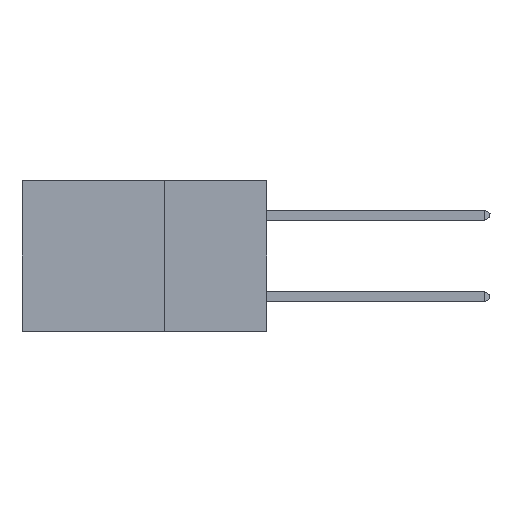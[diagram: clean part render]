
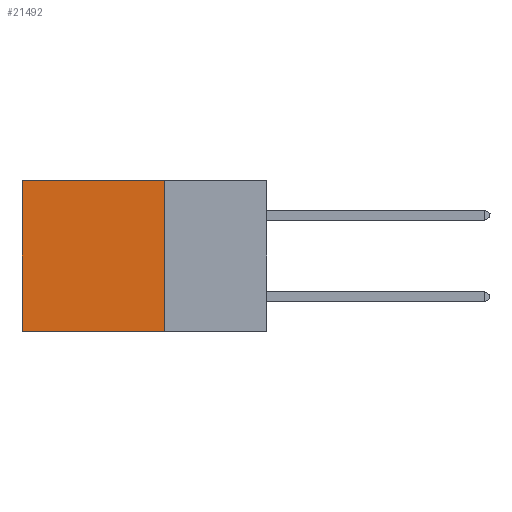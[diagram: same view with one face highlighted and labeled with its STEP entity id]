
A CAD part, left-side view. The second image highlights one B-rep face of the part: STEP entity #21492.
In plain terms, the highlighted planar face has unit normal (-1, 0, 0).
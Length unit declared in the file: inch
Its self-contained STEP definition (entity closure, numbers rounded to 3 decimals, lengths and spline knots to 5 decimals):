
#578 = CARTESIAN_POINT ( 'NONE',  ( 0.2875, 0.6, 0. ) ) ;
#723 = DIRECTION ( 'NONE',  ( 0., 0., -1. ) ) ;
#856 = PLANE ( 'NONE',  #13814 ) ;
#1374 = CARTESIAN_POINT ( 'NONE',  ( 0.2875, 0.6, 0. ) ) ;
#1841 = ORIENTED_EDGE ( 'NONE', *, *, #5590, .F. ) ;
#2267 = ORIENTED_EDGE ( 'NONE', *, *, #13636, .F. ) ;
#2281 = CARTESIAN_POINT ( 'NONE',  ( 0.2875, 0.25, -0.37 ) ) ;
#2628 = DIRECTION ( 'NONE',  ( 0., 0., -1. ) ) ;
#4693 = VERTEX_POINT ( 'NONE', #1374 ) ;
#5151 = LINE ( 'NONE', #16230, #18404 ) ;
#5344 = EDGE_CURVE ( 'NONE', #11775, #4693, #17282, .T. ) ;
#5590 = EDGE_CURVE ( 'NONE', #11775, #10790, #12466, .T. ) ;
#5889 = DIRECTION ( 'NONE',  ( 0., 0., -1. ) ) ;
#6041 = DIRECTION ( 'NONE',  ( 0., 1., 0. ) ) ;
#6664 = CARTESIAN_POINT ( 'NONE',  ( 0.2875, 0.6, -0.37 ) ) ;
#7104 = VECTOR ( 'NONE', #5889, 39.37008 ) ;
#7495 = ORIENTED_EDGE ( 'NONE', *, *, #19419, .T. ) ;
#7590 = EDGE_LOOP ( 'NONE', ( #7495, #2267, #1841, #22154 ) ) ;
#8167 = VECTOR ( 'NONE', #6041, 39.37008 ) ;
#10790 = VERTEX_POINT ( 'NONE', #2281 ) ;
#11775 = VERTEX_POINT ( 'NONE', #19070 ) ;
#12466 = LINE ( 'NONE', #20585, #16453 ) ;
#13069 = DIRECTION ( 'NONE',  ( 1., 0., 0. ) ) ;
#13541 = FACE_OUTER_BOUND ( 'NONE', #7590, .T. ) ;
#13636 = EDGE_CURVE ( 'NONE', #10790, #19724, #5151, .T. ) ;
#13814 = AXIS2_PLACEMENT_3D ( 'NONE', #21618, #13069, #2628 ) ;
#16230 = CARTESIAN_POINT ( 'NONE',  ( 0.2875, 0.25, -0.37 ) ) ;
#16453 = VECTOR ( 'NONE', #723, 39.37008 ) ;
#17282 = LINE ( 'NONE', #19344, #8167 ) ;
#17884 = DIRECTION ( 'NONE',  ( 0., 1., 0. ) ) ;
#18404 = VECTOR ( 'NONE', #17884, 39.37008 ) ;
#19070 = CARTESIAN_POINT ( 'NONE',  ( 0.2875, 0.25, 0. ) ) ;
#19344 = CARTESIAN_POINT ( 'NONE',  ( 0.2875, 0.25, 0. ) ) ;
#19419 = EDGE_CURVE ( 'NONE', #4693, #19724, #21356, .T. ) ;
#19724 = VERTEX_POINT ( 'NONE', #6664 ) ;
#20585 = CARTESIAN_POINT ( 'NONE',  ( 0.2875, 0.25, 0. ) ) ;
#21356 = LINE ( 'NONE', #578, #7104 ) ;
#21492 = ADVANCED_FACE ( 'NONE', ( #13541 ), #856, .F. ) ;
#21618 = CARTESIAN_POINT ( 'NONE',  ( 0.2875, 0.25, 0. ) ) ;
#22154 = ORIENTED_EDGE ( 'NONE', *, *, #5344, .T. ) ;
